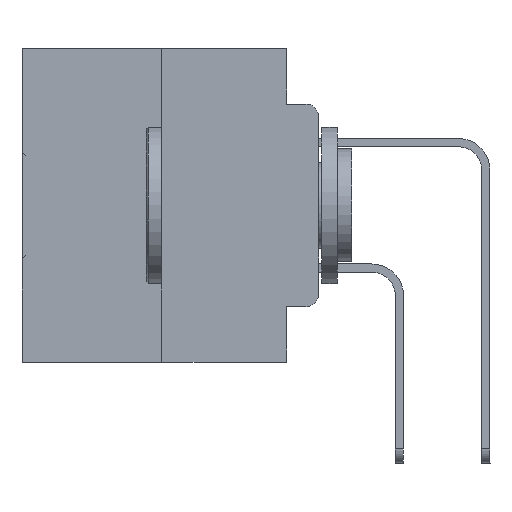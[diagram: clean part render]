
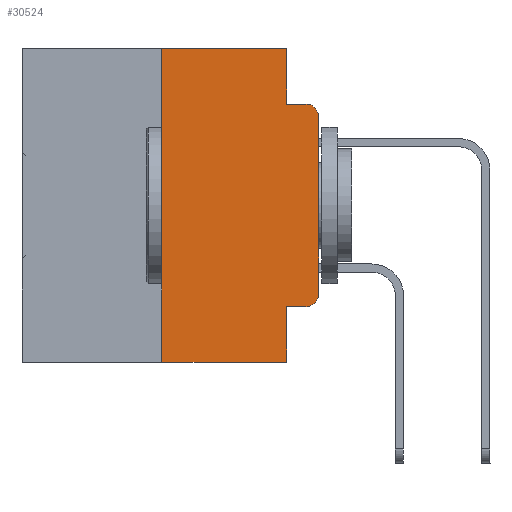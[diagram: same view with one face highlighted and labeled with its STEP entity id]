
A CAD part, left-side view. The second image highlights one B-rep face of the part: STEP entity #30524.
In plain terms, the highlighted planar face has unit normal (-1, 0, 0).
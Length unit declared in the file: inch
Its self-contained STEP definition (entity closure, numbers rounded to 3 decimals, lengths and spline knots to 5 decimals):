
#171 = CARTESIAN_POINT ( 'NONE',  ( 0., 0., 0. ) ) ;
#381 = ORIENTED_EDGE ( 'NONE', *, *, #28472, .T. ) ;
#627 = CARTESIAN_POINT ( 'NONE',  ( 0., 0.473, 0. ) ) ;
#1008 = VERTEX_POINT ( 'NONE', #15935 ) ;
#1603 = AXIS2_PLACEMENT_3D ( 'NONE', #21548, #5729, #24222 ) ;
#1778 = DIRECTION ( 'NONE',  ( -1., 0., 0. ) ) ;
#2828 = FACE_OUTER_BOUND ( 'NONE', #26652, .T. ) ;
#3049 = EDGE_CURVE ( 'NONE', #15066, #21938, #24016, .T. ) ;
#3319 = VECTOR ( 'NONE', #18781, 39.37008 ) ;
#3893 = ORIENTED_EDGE ( 'NONE', *, *, #10235, .T. ) ;
#3987 = VECTOR ( 'NONE', #19178, 39.37008 ) ;
#4162 = CARTESIAN_POINT ( 'NONE',  ( 0., 0.473, 0. ) ) ;
#4595 = LINE ( 'NONE', #4162, #11675 ) ;
#4874 = EDGE_CURVE ( 'NONE', #21938, #23381, #23058, .T. ) ;
#5348 = CARTESIAN_POINT ( 'NONE',  ( 0., 0., -0.1085 ) ) ;
#5360 = CARTESIAN_POINT ( 'NONE',  ( 0., 0.051, 0. ) ) ;
#5562 = ORIENTED_EDGE ( 'NONE', *, *, #12947, .F. ) ;
#5664 = LINE ( 'NONE', #19058, #3987 ) ;
#5729 = DIRECTION ( 'NONE',  ( -1., 0., 0. ) ) ;
#6972 = LINE ( 'NONE', #15261, #20194 ) ;
#8014 = DIRECTION ( 'NONE',  ( 0., 0., -1. ) ) ;
#8996 = VECTOR ( 'NONE', #23320, 39.37008 ) ;
#9068 = LINE ( 'NONE', #5360, #22293 ) ;
#9303 = ORIENTED_EDGE ( 'NONE', *, *, #12008, .T. ) ;
#9719 = CIRCLE ( 'NONE', #20234, 0.02 ) ;
#10235 = EDGE_CURVE ( 'NONE', #23871, #23381, #9719, .T. ) ;
#10239 = VERTEX_POINT ( 'NONE', #22902 ) ;
#10294 = LINE ( 'NONE', #32607, #24300 ) ;
#11333 = PLANE ( 'NONE',  #32920 ) ;
#11440 = DIRECTION ( 'NONE',  ( 0., 0., -1. ) ) ;
#11675 = VECTOR ( 'NONE', #17340, 39.37008 ) ;
#12008 = EDGE_CURVE ( 'NONE', #23588, #23871, #17405, .T. ) ;
#12199 = CARTESIAN_POINT ( 'NONE',  ( 0., 0.051, 0. ) ) ;
#12754 = CARTESIAN_POINT ( 'NONE',  ( 0., 0.051, -0.0885 ) ) ;
#12947 = EDGE_CURVE ( 'NONE', #1008, #15066, #4595, .T. ) ;
#14768 = CARTESIAN_POINT ( 'NONE',  ( 0., 0., -0.3915 ) ) ;
#15066 = VERTEX_POINT ( 'NONE', #16440 ) ;
#15261 = CARTESIAN_POINT ( 'NONE',  ( 0., 0.051, -0.4115 ) ) ;
#15626 = VERTEX_POINT ( 'NONE', #31699 ) ;
#15935 = CARTESIAN_POINT ( 'NONE',  ( 0., 0.25, 0. ) ) ;
#16440 = CARTESIAN_POINT ( 'NONE',  ( 0., 0.051, 0. ) ) ;
#17017 = DIRECTION ( 'NONE',  ( 0., 0., 1. ) ) ;
#17340 = DIRECTION ( 'NONE',  ( 0., -1., 0. ) ) ;
#17405 = LINE ( 'NONE', #171, #3319 ) ;
#17677 = CARTESIAN_POINT ( 'NONE',  ( 0., 0.02, -0.1085 ) ) ;
#17875 = DIRECTION ( 'NONE',  ( 0., -1., 0. ) ) ;
#18781 = DIRECTION ( 'NONE',  ( 0., 0., 1. ) ) ;
#19058 = CARTESIAN_POINT ( 'NONE',  ( 0., 0.473, -0.5 ) ) ;
#19178 = DIRECTION ( 'NONE',  ( 0., -1., 0. ) ) ;
#20194 = VECTOR ( 'NONE', #17875, 39.37008 ) ;
#20234 = AXIS2_PLACEMENT_3D ( 'NONE', #17677, #1778, #20335 ) ;
#20335 = DIRECTION ( 'NONE',  ( 0., 0., -1. ) ) ;
#21271 = ORIENTED_EDGE ( 'NONE', *, *, #33617, .F. ) ;
#21548 = CARTESIAN_POINT ( 'NONE',  ( 0., 0.02, -0.3915 ) ) ;
#21938 = VERTEX_POINT ( 'NONE', #28723 ) ;
#22293 = VECTOR ( 'NONE', #8014, 39.37008 ) ;
#22500 = VERTEX_POINT ( 'NONE', #25718 ) ;
#22865 = VERTEX_POINT ( 'NONE', #27507 ) ;
#22902 = CARTESIAN_POINT ( 'NONE',  ( 0., 0.02, -0.4115 ) ) ;
#22956 = ORIENTED_EDGE ( 'NONE', *, *, #34038, .T. ) ;
#23058 = LINE ( 'NONE', #12754, #8996 ) ;
#23320 = DIRECTION ( 'NONE',  ( 0., -1., 0. ) ) ;
#23381 = VERTEX_POINT ( 'NONE', #27140 ) ;
#23588 = VERTEX_POINT ( 'NONE', #14768 ) ;
#23871 = VERTEX_POINT ( 'NONE', #5348 ) ;
#24016 = LINE ( 'NONE', #12199, #30068 ) ;
#24222 = DIRECTION ( 'NONE',  ( 0., 0., -1. ) ) ;
#24300 = VECTOR ( 'NONE', #17017, 39.37008 ) ;
#24981 = ORIENTED_EDGE ( 'NONE', *, *, #4874, .F. ) ;
#25692 = CIRCLE ( 'NONE', #1603, 0.02 ) ;
#25718 = CARTESIAN_POINT ( 'NONE',  ( 0., 0.051, -0.4115 ) ) ;
#26562 = DIRECTION ( 'NONE',  ( 0., 0., -1. ) ) ;
#26652 = EDGE_LOOP ( 'NONE', ( #9303, #3893, #24981, #32633, #5562, #21271, #22956, #32125, #33736, #381 ) ) ;
#27140 = CARTESIAN_POINT ( 'NONE',  ( 0., 0.02, -0.0885 ) ) ;
#27148 = DIRECTION ( 'NONE',  ( 1., 0., 0. ) ) ;
#27507 = CARTESIAN_POINT ( 'NONE',  ( 0., 0.25, -0.5 ) ) ;
#28472 = EDGE_CURVE ( 'NONE', #10239, #23588, #25692, .T. ) ;
#28723 = CARTESIAN_POINT ( 'NONE',  ( 0., 0.051, -0.0885 ) ) ;
#30068 = VECTOR ( 'NONE', #26562, 39.37008 ) ;
#30177 = EDGE_CURVE ( 'NONE', #22500, #10239, #6972, .T. ) ;
#30524 = ADVANCED_FACE ( 'NONE', ( #2828 ), #11333, .F. ) ;
#31699 = CARTESIAN_POINT ( 'NONE',  ( 0., 0.051, -0.5 ) ) ;
#31899 = EDGE_CURVE ( 'NONE', #22500, #15626, #9068, .T. ) ;
#32125 = ORIENTED_EDGE ( 'NONE', *, *, #31899, .F. ) ;
#32607 = CARTESIAN_POINT ( 'NONE',  ( 0., 0.25, 0. ) ) ;
#32633 = ORIENTED_EDGE ( 'NONE', *, *, #3049, .F. ) ;
#32920 = AXIS2_PLACEMENT_3D ( 'NONE', #627, #27148, #11440 ) ;
#33617 = EDGE_CURVE ( 'NONE', #22865, #1008, #10294, .T. ) ;
#33736 = ORIENTED_EDGE ( 'NONE', *, *, #30177, .T. ) ;
#34038 = EDGE_CURVE ( 'NONE', #22865, #15626, #5664, .T. ) ;
